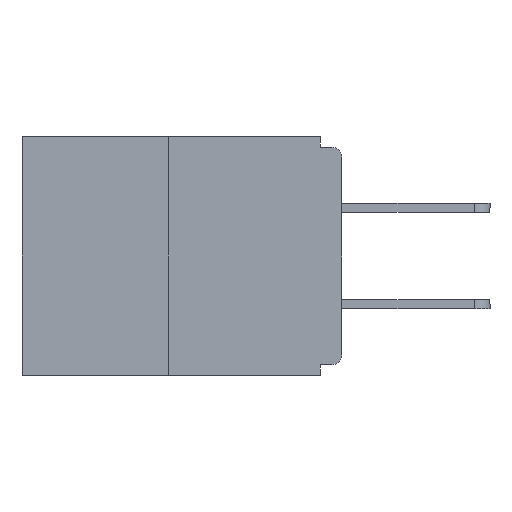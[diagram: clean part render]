
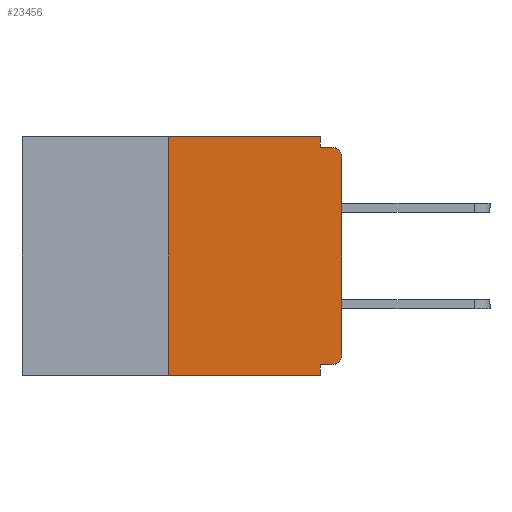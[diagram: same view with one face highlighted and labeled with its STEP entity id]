
A CAD part, left-side view. The second image highlights one B-rep face of the part: STEP entity #23456.
In plain terms, the highlighted planar face has unit normal (-1, 0, 0).
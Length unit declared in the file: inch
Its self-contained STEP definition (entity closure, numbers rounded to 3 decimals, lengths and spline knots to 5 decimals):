
#95 = EDGE_CURVE ( 'NONE', #1303, #1132, #14968, .T. ) ;
#290 = CARTESIAN_POINT ( 'NONE',  ( 0., 0.031, 0. ) ) ;
#430 = DIRECTION ( 'NONE',  ( 0., 0., -1. ) ) ;
#622 = CARTESIAN_POINT ( 'NONE',  ( 0., 0.031, -0.343 ) ) ;
#910 = ORIENTED_EDGE ( 'NONE', *, *, #20184, .F. ) ;
#1106 = AXIS2_PLACEMENT_3D ( 'NONE', #19841, #24106, #430 ) ;
#1132 = VERTEX_POINT ( 'NONE', #20806 ) ;
#1303 = VERTEX_POINT ( 'NONE', #22909 ) ;
#1590 = CARTESIAN_POINT ( 'NONE',  ( 0., 0.015, -0.328 ) ) ;
#2417 = LINE ( 'NONE', #9387, #15414 ) ;
#2897 = DIRECTION ( 'NONE',  ( 0., 0., -1. ) ) ;
#2999 = ORIENTED_EDGE ( 'NONE', *, *, #22678, .T. ) ;
#4027 = EDGE_CURVE ( 'NONE', #12650, #9093, #13104, .T. ) ;
#4676 = ORIENTED_EDGE ( 'NONE', *, *, #23884, .T. ) ;
#4776 = VECTOR ( 'NONE', #20085, 39.37008 ) ;
#5248 = CARTESIAN_POINT ( 'NONE',  ( 0., 0.25, 0. ) ) ;
#5885 = DIRECTION ( 'NONE',  ( 0., -1., 0. ) ) ;
#5947 = DIRECTION ( 'NONE',  ( 0., 0., -1. ) ) ;
#6117 = ORIENTED_EDGE ( 'NONE', *, *, #10910, .T. ) ;
#6696 = CARTESIAN_POINT ( 'NONE',  ( 0., 0.015, -0.313 ) ) ;
#6995 = EDGE_LOOP ( 'NONE', ( #22884, #910, #2999, #20697, #7901, #8861, #4676, #6117, #14096, #10099 ) ) ;
#7354 = EDGE_CURVE ( 'NONE', #9093, #18943, #2417, .T. ) ;
#7815 = VECTOR ( 'NONE', #19852, 39.37008 ) ;
#7901 = ORIENTED_EDGE ( 'NONE', *, *, #4027, .F. ) ;
#8632 = CARTESIAN_POINT ( 'NONE',  ( 0., 0.46, 0. ) ) ;
#8861 = ORIENTED_EDGE ( 'NONE', *, *, #25584, .T. ) ;
#9093 = VERTEX_POINT ( 'NONE', #9995 ) ;
#9387 = CARTESIAN_POINT ( 'NONE',  ( 0., 0.031, -0.343 ) ) ;
#9454 = CARTESIAN_POINT ( 'NONE',  ( 0., 0.25, 0. ) ) ;
#9495 = LINE ( 'NONE', #15427, #24023 ) ;
#9995 = CARTESIAN_POINT ( 'NONE',  ( 0., 0.031, -0.328 ) ) ;
#10036 = PLANE ( 'NONE',  #1106 ) ;
#10099 = ORIENTED_EDGE ( 'NONE', *, *, #18037, .F. ) ;
#10685 = CARTESIAN_POINT ( 'NONE',  ( 0., 0., -0.015 ) ) ;
#10779 = DIRECTION ( 'NONE',  ( -1., 0., 0. ) ) ;
#10790 = VECTOR ( 'NONE', #23288, 39.37008 ) ;
#10894 = LINE ( 'NONE', #19615, #12764 ) ;
#10910 = EDGE_CURVE ( 'NONE', #13963, #1132, #13378, .T. ) ;
#11396 = DIRECTION ( 'NONE',  ( 0., 0., -1. ) ) ;
#12246 = LINE ( 'NONE', #16068, #4776 ) ;
#12650 = VERTEX_POINT ( 'NONE', #1590 ) ;
#12764 = VECTOR ( 'NONE', #5947, 39.37008 ) ;
#12824 = VECTOR ( 'NONE', #24504, 39.37008 ) ;
#13104 = LINE ( 'NONE', #19451, #7815 ) ;
#13116 = EDGE_CURVE ( 'NONE', #25012, #22452, #19750, .T. ) ;
#13279 = CARTESIAN_POINT ( 'NONE',  ( 0., 0., -0.313 ) ) ;
#13378 = CIRCLE ( 'NONE', #14002, 0.015 ) ;
#13963 = VERTEX_POINT ( 'NONE', #17758 ) ;
#14002 = AXIS2_PLACEMENT_3D ( 'NONE', #16896, #10779, #2897 ) ;
#14096 = ORIENTED_EDGE ( 'NONE', *, *, #95, .F. ) ;
#14528 = DIRECTION ( 'NONE',  ( 0., -1., 0. ) ) ;
#14767 = DIRECTION ( 'NONE',  ( 0., 0., -1. ) ) ;
#14968 = LINE ( 'NONE', #10685, #12824 ) ;
#15414 = VECTOR ( 'NONE', #11396, 39.37008 ) ;
#15427 = CARTESIAN_POINT ( 'NONE',  ( 0., 0.46, -0.343 ) ) ;
#16068 = CARTESIAN_POINT ( 'NONE',  ( 0., 0., 0. ) ) ;
#16668 = DIRECTION ( 'NONE',  ( -1., 0., 0. ) ) ;
#16896 = CARTESIAN_POINT ( 'NONE',  ( 0., 0.015, -0.03 ) ) ;
#17758 = CARTESIAN_POINT ( 'NONE',  ( 0., 0., -0.03 ) ) ;
#17784 = FACE_OUTER_BOUND ( 'NONE', #6995, .T. ) ;
#18037 = EDGE_CURVE ( 'NONE', #22452, #1303, #10894, .T. ) ;
#18492 = LINE ( 'NONE', #9454, #10790 ) ;
#18943 = VERTEX_POINT ( 'NONE', #622 ) ;
#19451 = CARTESIAN_POINT ( 'NONE',  ( 0., 0., -0.328 ) ) ;
#19473 = CARTESIAN_POINT ( 'NONE',  ( 0., 0.25, -0.343 ) ) ;
#19615 = CARTESIAN_POINT ( 'NONE',  ( 0., 0.031, 0. ) ) ;
#19750 = LINE ( 'NONE', #8632, #20038 ) ;
#19841 = CARTESIAN_POINT ( 'NONE',  ( 0., 0.46, 0. ) ) ;
#19852 = DIRECTION ( 'NONE',  ( 0., 1., 0. ) ) ;
#20038 = VECTOR ( 'NONE', #14528, 39.37008 ) ;
#20085 = DIRECTION ( 'NONE',  ( 0., 0., 1. ) ) ;
#20184 = EDGE_CURVE ( 'NONE', #22365, #25012, #18492, .T. ) ;
#20697 = ORIENTED_EDGE ( 'NONE', *, *, #7354, .F. ) ;
#20806 = CARTESIAN_POINT ( 'NONE',  ( 0., 0.015, -0.015 ) ) ;
#22334 = VERTEX_POINT ( 'NONE', #13279 ) ;
#22365 = VERTEX_POINT ( 'NONE', #19473 ) ;
#22452 = VERTEX_POINT ( 'NONE', #290 ) ;
#22495 = AXIS2_PLACEMENT_3D ( 'NONE', #6696, #16668, #14767 ) ;
#22678 = EDGE_CURVE ( 'NONE', #22365, #18943, #9495, .T. ) ;
#22884 = ORIENTED_EDGE ( 'NONE', *, *, #13116, .F. ) ;
#22909 = CARTESIAN_POINT ( 'NONE',  ( 0., 0.031, -0.015 ) ) ;
#23288 = DIRECTION ( 'NONE',  ( 0., 0., 1. ) ) ;
#23456 = ADVANCED_FACE ( 'NONE', ( #17784 ), #10036, .F. ) ;
#23884 = EDGE_CURVE ( 'NONE', #22334, #13963, #12246, .T. ) ;
#24023 = VECTOR ( 'NONE', #5885, 39.37008 ) ;
#24106 = DIRECTION ( 'NONE',  ( 1., 0., 0. ) ) ;
#24504 = DIRECTION ( 'NONE',  ( 0., -1., 0. ) ) ;
#24789 = CIRCLE ( 'NONE', #22495, 0.015 ) ;
#25012 = VERTEX_POINT ( 'NONE', #5248 ) ;
#25584 = EDGE_CURVE ( 'NONE', #12650, #22334, #24789, .T. ) ;
